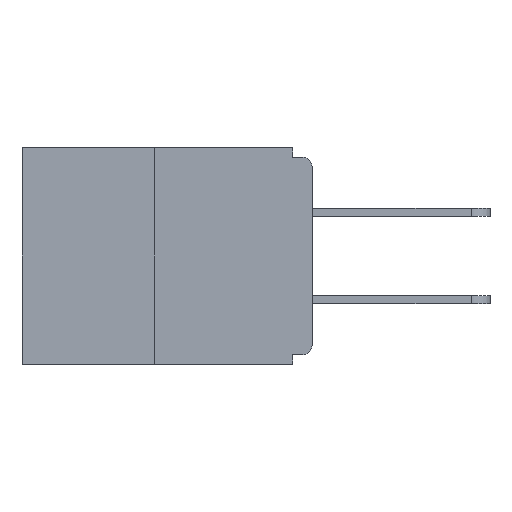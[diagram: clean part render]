
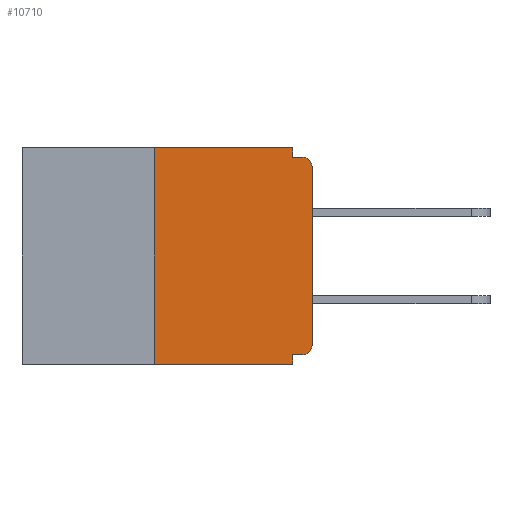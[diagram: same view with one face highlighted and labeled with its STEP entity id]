
A CAD part, left-side view. The second image highlights one B-rep face of the part: STEP entity #10710.
In plain terms, the highlighted planar face has unit normal (-1, 0, 0).
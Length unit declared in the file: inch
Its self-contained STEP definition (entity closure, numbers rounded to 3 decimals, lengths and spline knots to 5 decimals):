
#20 = CARTESIAN_POINT ( 'NONE',  ( 0., 0., -0.328 ) ) ;
#262 = EDGE_CURVE ( 'NONE', #12682, #21692, #14190, .T. ) ;
#564 = LINE ( 'NONE', #10923, #15690 ) ;
#633 = EDGE_CURVE ( 'NONE', #21102, #10780, #8898, .T. ) ;
#647 = AXIS2_PLACEMENT_3D ( 'NONE', #1773, #7747, #21583 ) ;
#721 = EDGE_CURVE ( 'NONE', #23799, #21039, #7325, .T. ) ;
#851 = DIRECTION ( 'NONE',  ( 0., -1., 0. ) ) ;
#1139 = AXIS2_PLACEMENT_3D ( 'NONE', #22813, #10987, #17243 ) ;
#1679 = EDGE_CURVE ( 'NONE', #16904, #6732, #22174, .T. ) ;
#1773 = CARTESIAN_POINT ( 'NONE',  ( 0., 0.015, -0.313 ) ) ;
#1877 = CARTESIAN_POINT ( 'NONE',  ( 0., 0., -0.03 ) ) ;
#2133 = VECTOR ( 'NONE', #5514, 39.37008 ) ;
#2513 = CARTESIAN_POINT ( 'NONE',  ( 0., 0., -0.015 ) ) ;
#2660 = CARTESIAN_POINT ( 'NONE',  ( 0., 0.015, -0.015 ) ) ;
#2802 = LINE ( 'NONE', #20, #24511 ) ;
#3531 = EDGE_LOOP ( 'NONE', ( #14219, #23201, #5109, #19020, #16369, #21808, #20544, #17617, #18579, #5169 ) ) ;
#5109 = ORIENTED_EDGE ( 'NONE', *, *, #13813, .T. ) ;
#5169 = ORIENTED_EDGE ( 'NONE', *, *, #1679, .F. ) ;
#5514 = DIRECTION ( 'NONE',  ( 0., 0., 1. ) ) ;
#5816 = EDGE_CURVE ( 'NONE', #21692, #16904, #25423, .T. ) ;
#5826 = CARTESIAN_POINT ( 'NONE',  ( 0., 0., -0.313 ) ) ;
#6060 = CARTESIAN_POINT ( 'NONE',  ( 0., 0., 0. ) ) ;
#6732 = VERTEX_POINT ( 'NONE', #16217 ) ;
#6761 = VERTEX_POINT ( 'NONE', #2660 ) ;
#7188 = FACE_OUTER_BOUND ( 'NONE', #3531, .T. ) ;
#7216 = DIRECTION ( 'NONE',  ( 0., 0., -1. ) ) ;
#7325 = LINE ( 'NONE', #6060, #20951 ) ;
#7488 = LINE ( 'NONE', #2513, #10308 ) ;
#7517 = CARTESIAN_POINT ( 'NONE',  ( 0., 0.46, 0. ) ) ;
#7731 = PLANE ( 'NONE',  #16530 ) ;
#7747 = DIRECTION ( 'NONE',  ( -1., 0., 0. ) ) ;
#7817 = DIRECTION ( 'NONE',  ( 0., 0., -1. ) ) ;
#8898 = LINE ( 'NONE', #15454, #15992 ) ;
#9172 = CARTESIAN_POINT ( 'NONE',  ( 0., 0.25, -0.343 ) ) ;
#10075 = CARTESIAN_POINT ( 'NONE',  ( 0., 0.031, -0.343 ) ) ;
#10308 = VECTOR ( 'NONE', #24261, 39.37008 ) ;
#10710 = ADVANCED_FACE ( 'NONE', ( #7188 ), #7731, .F. ) ;
#10780 = VERTEX_POINT ( 'NONE', #10075 ) ;
#10923 = CARTESIAN_POINT ( 'NONE',  ( 0., 0.46, -0.343 ) ) ;
#10987 = DIRECTION ( 'NONE',  ( -1., 0., 0. ) ) ;
#11191 = VERTEX_POINT ( 'NONE', #13174 ) ;
#11716 = CARTESIAN_POINT ( 'NONE',  ( 0., 0.46, 0. ) ) ;
#12319 = EDGE_CURVE ( 'NONE', #21039, #6761, #20749, .T. ) ;
#12682 = VERTEX_POINT ( 'NONE', #9172 ) ;
#13174 = CARTESIAN_POINT ( 'NONE',  ( 0., 0.015, -0.328 ) ) ;
#13813 = EDGE_CURVE ( 'NONE', #12682, #10780, #564, .T. ) ;
#14190 = LINE ( 'NONE', #25217, #2133 ) ;
#14219 = ORIENTED_EDGE ( 'NONE', *, *, #5816, .F. ) ;
#15454 = CARTESIAN_POINT ( 'NONE',  ( 0., 0.031, -0.343 ) ) ;
#15646 = DIRECTION ( 'NONE',  ( 1., 0., 0. ) ) ;
#15690 = VECTOR ( 'NONE', #851, 39.37008 ) ;
#15843 = DIRECTION ( 'NONE',  ( 0., 1., 0. ) ) ;
#15992 = VECTOR ( 'NONE', #25133, 39.37008 ) ;
#16168 = CARTESIAN_POINT ( 'NONE',  ( 0., 0.25, 0. ) ) ;
#16217 = CARTESIAN_POINT ( 'NONE',  ( 0., 0.031, -0.015 ) ) ;
#16248 = VECTOR ( 'NONE', #7216, 39.37008 ) ;
#16369 = ORIENTED_EDGE ( 'NONE', *, *, #23731, .F. ) ;
#16530 = AXIS2_PLACEMENT_3D ( 'NONE', #11716, #15646, #7817 ) ;
#16904 = VERTEX_POINT ( 'NONE', #22556 ) ;
#17243 = DIRECTION ( 'NONE',  ( 0., 0., -1. ) ) ;
#17617 = ORIENTED_EDGE ( 'NONE', *, *, #12319, .T. ) ;
#18579 = ORIENTED_EDGE ( 'NONE', *, *, #24413, .F. ) ;
#19020 = ORIENTED_EDGE ( 'NONE', *, *, #633, .F. ) ;
#19111 = CARTESIAN_POINT ( 'NONE',  ( 0., 0.031, 0. ) ) ;
#20544 = ORIENTED_EDGE ( 'NONE', *, *, #721, .T. ) ;
#20723 = VECTOR ( 'NONE', #21532, 39.37008 ) ;
#20749 = CIRCLE ( 'NONE', #1139, 0.015 ) ;
#20951 = VECTOR ( 'NONE', #21730, 39.37008 ) ;
#21039 = VERTEX_POINT ( 'NONE', #1877 ) ;
#21102 = VERTEX_POINT ( 'NONE', #25536 ) ;
#21532 = DIRECTION ( 'NONE',  ( 0., -1., 0. ) ) ;
#21583 = DIRECTION ( 'NONE',  ( 0., 0., -1. ) ) ;
#21692 = VERTEX_POINT ( 'NONE', #16168 ) ;
#21730 = DIRECTION ( 'NONE',  ( 0., 0., 1. ) ) ;
#21808 = ORIENTED_EDGE ( 'NONE', *, *, #23721, .T. ) ;
#22174 = LINE ( 'NONE', #19111, #16248 ) ;
#22556 = CARTESIAN_POINT ( 'NONE',  ( 0., 0.031, 0. ) ) ;
#22813 = CARTESIAN_POINT ( 'NONE',  ( 0., 0.015, -0.03 ) ) ;
#23201 = ORIENTED_EDGE ( 'NONE', *, *, #262, .F. ) ;
#23721 = EDGE_CURVE ( 'NONE', #11191, #23799, #24817, .T. ) ;
#23731 = EDGE_CURVE ( 'NONE', #11191, #21102, #2802, .T. ) ;
#23799 = VERTEX_POINT ( 'NONE', #5826 ) ;
#24261 = DIRECTION ( 'NONE',  ( 0., -1., 0. ) ) ;
#24413 = EDGE_CURVE ( 'NONE', #6732, #6761, #7488, .T. ) ;
#24511 = VECTOR ( 'NONE', #15843, 39.37008 ) ;
#24817 = CIRCLE ( 'NONE', #647, 0.015 ) ;
#25133 = DIRECTION ( 'NONE',  ( 0., 0., -1. ) ) ;
#25217 = CARTESIAN_POINT ( 'NONE',  ( 0., 0.25, 0. ) ) ;
#25423 = LINE ( 'NONE', #7517, #20723 ) ;
#25536 = CARTESIAN_POINT ( 'NONE',  ( 0., 0.031, -0.328 ) ) ;
